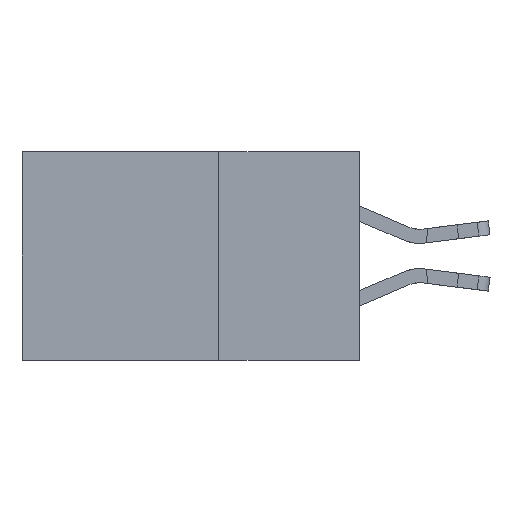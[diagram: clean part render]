
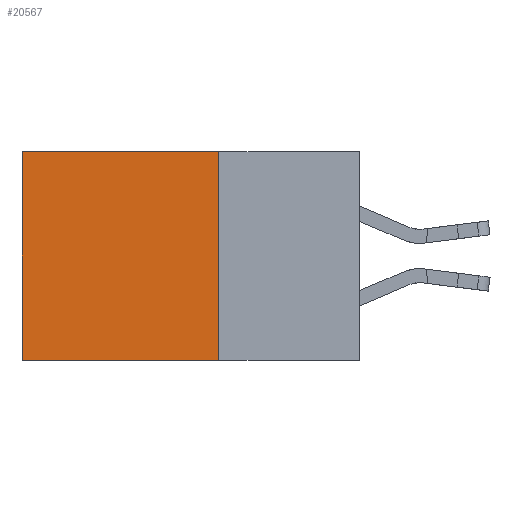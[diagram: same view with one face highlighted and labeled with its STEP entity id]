
A CAD part, left-side view. The second image highlights one B-rep face of the part: STEP entity #20567.
In plain terms, the highlighted planar face has unit normal (-1, 0, 0).
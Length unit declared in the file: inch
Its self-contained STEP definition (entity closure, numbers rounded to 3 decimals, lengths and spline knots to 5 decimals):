
#543 = VERTEX_POINT ( 'NONE', #6931 ) ;
#2960 = LINE ( 'NONE', #15495, #11016 ) ;
#3593 = DIRECTION ( 'NONE',  ( 1., 0., 0. ) ) ;
#3856 = CARTESIAN_POINT ( 'NONE',  ( 0.2875, 0.25, -0.37 ) ) ;
#5031 = EDGE_CURVE ( 'NONE', #543, #10712, #20253, .T. ) ;
#5521 = CARTESIAN_POINT ( 'NONE',  ( 0.2875, 0.25, 0. ) ) ;
#5525 = VECTOR ( 'NONE', #19955, 39.37008 ) ;
#6828 = DIRECTION ( 'NONE',  ( 0., 0., -1. ) ) ;
#6931 = CARTESIAN_POINT ( 'NONE',  ( 0.2875, 0.25, -0.37 ) ) ;
#7137 = DIRECTION ( 'NONE',  ( 0., 1., 0. ) ) ;
#7180 = VERTEX_POINT ( 'NONE', #10125 ) ;
#7330 = FACE_OUTER_BOUND ( 'NONE', #16732, .T. ) ;
#8242 = ORIENTED_EDGE ( 'NONE', *, *, #18395, .T. ) ;
#8757 = ORIENTED_EDGE ( 'NONE', *, *, #8930, .T. ) ;
#8930 = EDGE_CURVE ( 'NONE', #9876, #10712, #11418, .T. ) ;
#9795 = ORIENTED_EDGE ( 'NONE', *, *, #17479, .F. ) ;
#9876 = VERTEX_POINT ( 'NONE', #20479 ) ;
#10095 = CARTESIAN_POINT ( 'NONE',  ( 0.2875, 0.25, 0. ) ) ;
#10125 = CARTESIAN_POINT ( 'NONE',  ( 0.2875, 0.25, 0. ) ) ;
#10712 = VERTEX_POINT ( 'NONE', #15537 ) ;
#11016 = VECTOR ( 'NONE', #18598, 39.37008 ) ;
#11418 = LINE ( 'NONE', #15969, #18094 ) ;
#13001 = AXIS2_PLACEMENT_3D ( 'NONE', #10095, #3593, #6828 ) ;
#13453 = ORIENTED_EDGE ( 'NONE', *, *, #5031, .F. ) ;
#14182 = DIRECTION ( 'NONE',  ( 0., 0., -1. ) ) ;
#15495 = CARTESIAN_POINT ( 'NONE',  ( 0.2875, 0.25, 0. ) ) ;
#15537 = CARTESIAN_POINT ( 'NONE',  ( 0.2875, 0.6, -0.37 ) ) ;
#15969 = CARTESIAN_POINT ( 'NONE',  ( 0.2875, 0.6, 0. ) ) ;
#16732 = EDGE_LOOP ( 'NONE', ( #8757, #13453, #9795, #8242 ) ) ;
#16886 = LINE ( 'NONE', #5521, #20157 ) ;
#17479 = EDGE_CURVE ( 'NONE', #7180, #543, #2960, .T. ) ;
#18094 = VECTOR ( 'NONE', #14182, 39.37008 ) ;
#18393 = PLANE ( 'NONE',  #13001 ) ;
#18395 = EDGE_CURVE ( 'NONE', #7180, #9876, #16886, .T. ) ;
#18598 = DIRECTION ( 'NONE',  ( 0., 0., -1. ) ) ;
#19955 = DIRECTION ( 'NONE',  ( 0., 1., 0. ) ) ;
#20157 = VECTOR ( 'NONE', #7137, 39.37008 ) ;
#20253 = LINE ( 'NONE', #3856, #5525 ) ;
#20479 = CARTESIAN_POINT ( 'NONE',  ( 0.2875, 0.6, 0. ) ) ;
#20567 = ADVANCED_FACE ( 'NONE', ( #7330 ), #18393, .F. ) ;
